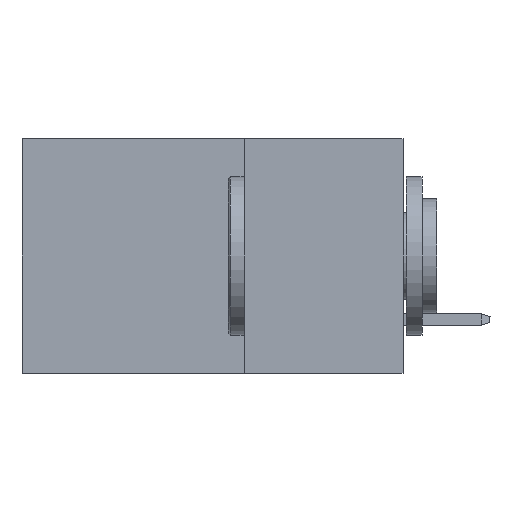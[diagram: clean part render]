
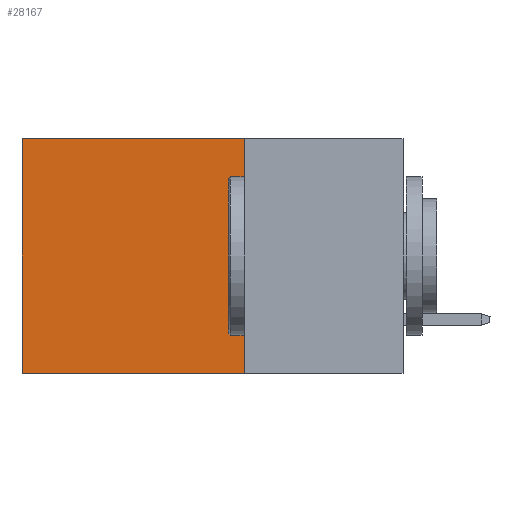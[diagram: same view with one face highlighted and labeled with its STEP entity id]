
A CAD part, left-side view. The second image highlights one B-rep face of the part: STEP entity #28167.
In plain terms, the highlighted planar face has unit normal (-1, 0, 0).
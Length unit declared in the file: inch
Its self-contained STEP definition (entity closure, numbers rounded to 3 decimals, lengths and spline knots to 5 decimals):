
#1291 = LINE ( 'NONE', #19295, #1296 ) ;
#1296 = VECTOR ( 'NONE', #4148, 39.37008 ) ;
#2812 = DIRECTION ( 'NONE',  ( 1., 0., 0. ) ) ;
#3098 = ORIENTED_EDGE ( 'NONE', *, *, #9355, .F. ) ;
#4017 = LINE ( 'NONE', #8683, #27907 ) ;
#4148 = DIRECTION ( 'NONE',  ( 0., 1., 0. ) ) ;
#5096 = VERTEX_POINT ( 'NONE', #27501 ) ;
#5176 = DIRECTION ( 'NONE',  ( 0., 0., -1. ) ) ;
#5666 = CARTESIAN_POINT ( 'NONE',  ( 0.2875, 0.6, 0. ) ) ;
#7459 = PLANE ( 'NONE',  #16349 ) ;
#7626 = DIRECTION ( 'NONE',  ( 0., 0., -1. ) ) ;
#8683 = CARTESIAN_POINT ( 'NONE',  ( 0.2875, 0.25, -0.37 ) ) ;
#8815 = DIRECTION ( 'NONE',  ( 0., 0., -1. ) ) ;
#9355 = EDGE_CURVE ( 'NONE', #5096, #29342, #4017, .T. ) ;
#9779 = EDGE_CURVE ( 'NONE', #27573, #22393, #1291, .T. ) ;
#10022 = ORIENTED_EDGE ( 'NONE', *, *, #9779, .T. ) ;
#13323 = LINE ( 'NONE', #23502, #28917 ) ;
#13843 = EDGE_LOOP ( 'NONE', ( #15316, #3098, #23995, #10022 ) ) ;
#15316 = ORIENTED_EDGE ( 'NONE', *, *, #32589, .T. ) ;
#16349 = AXIS2_PLACEMENT_3D ( 'NONE', #22806, #2812, #7626 ) ;
#19295 = CARTESIAN_POINT ( 'NONE',  ( 0.2875, 0.25, 0. ) ) ;
#20319 = LINE ( 'NONE', #5666, #26610 ) ;
#21265 = EDGE_CURVE ( 'NONE', #27573, #5096, #13323, .T. ) ;
#22393 = VERTEX_POINT ( 'NONE', #26525 ) ;
#22806 = CARTESIAN_POINT ( 'NONE',  ( 0.2875, 0.25, 0. ) ) ;
#23502 = CARTESIAN_POINT ( 'NONE',  ( 0.2875, 0.25, 0. ) ) ;
#23995 = ORIENTED_EDGE ( 'NONE', *, *, #21265, .F. ) ;
#26525 = CARTESIAN_POINT ( 'NONE',  ( 0.2875, 0.6, 0. ) ) ;
#26610 = VECTOR ( 'NONE', #5176, 39.37008 ) ;
#27501 = CARTESIAN_POINT ( 'NONE',  ( 0.2875, 0.25, -0.37 ) ) ;
#27573 = VERTEX_POINT ( 'NONE', #29575 ) ;
#27907 = VECTOR ( 'NONE', #29698, 39.37008 ) ;
#28167 = ADVANCED_FACE ( 'NONE', ( #28303 ), #7459, .F. ) ;
#28303 = FACE_OUTER_BOUND ( 'NONE', #13843, .T. ) ;
#28917 = VECTOR ( 'NONE', #8815, 39.37008 ) ;
#29038 = CARTESIAN_POINT ( 'NONE',  ( 0.2875, 0.6, -0.37 ) ) ;
#29342 = VERTEX_POINT ( 'NONE', #29038 ) ;
#29575 = CARTESIAN_POINT ( 'NONE',  ( 0.2875, 0.25, 0. ) ) ;
#29698 = DIRECTION ( 'NONE',  ( 0., 1., 0. ) ) ;
#32589 = EDGE_CURVE ( 'NONE', #22393, #29342, #20319, .T. ) ;
